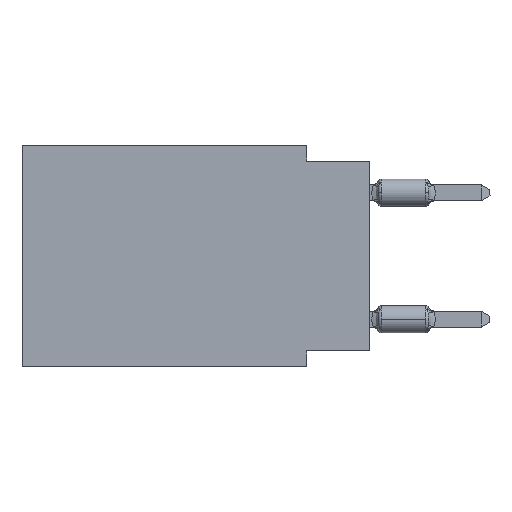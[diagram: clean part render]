
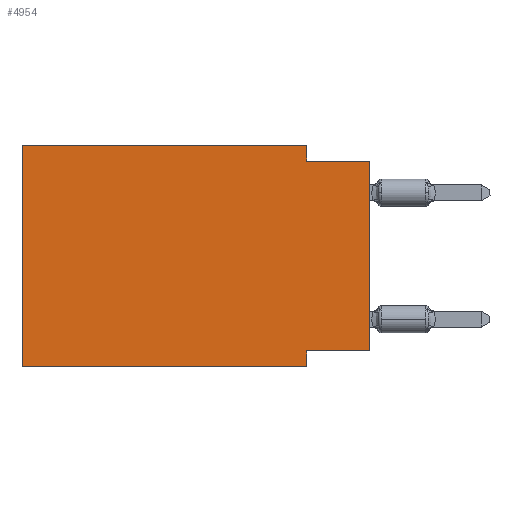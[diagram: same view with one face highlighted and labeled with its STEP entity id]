
A CAD part, left-side view. The second image highlights one B-rep face of the part: STEP entity #4954.
In plain terms, the highlighted planar face has unit normal (-1, 0, 0).
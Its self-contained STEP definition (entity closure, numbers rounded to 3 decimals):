
#300 = ORIENTED_EDGE ( 'NONE', *, *, #9761, .F. ) ;
#511 = CARTESIAN_POINT ( 'NONE',  ( 0., 2.54, 0. ) ) ;
#839 = ORIENTED_EDGE ( 'NONE', *, *, #12139, .T. ) ;
#884 = DIRECTION ( 'NONE',  ( 1., 0., 0. ) ) ;
#1540 = VECTOR ( 'NONE', #4809, 1000. ) ;
#1680 = ORIENTED_EDGE ( 'NONE', *, *, #12162, .F. ) ;
#1848 = PLANE ( 'NONE',  #8297 ) ;
#2168 = CARTESIAN_POINT ( 'NONE',  ( 0., 0., -8.255 ) ) ;
#2291 = VERTEX_POINT ( 'NONE', #4083 ) ;
#2313 = LINE ( 'NONE', #2168, #4158 ) ;
#2399 = DIRECTION ( 'NONE',  ( 0., 0., 1. ) ) ;
#2485 = DIRECTION ( 'NONE',  ( 0., -1., 0. ) ) ;
#2576 = LINE ( 'NONE', #3664, #7910 ) ;
#2777 = CARTESIAN_POINT ( 'NONE',  ( 0., 2.54, 0. ) ) ;
#3143 = VERTEX_POINT ( 'NONE', #5283 ) ;
#3512 = CARTESIAN_POINT ( 'NONE',  ( 0., 2.54, -8.89 ) ) ;
#3590 = EDGE_CURVE ( 'NONE', #2291, #4291, #6506, .T. ) ;
#3664 = CARTESIAN_POINT ( 'NONE',  ( 0., 13.97, -8.89 ) ) ;
#4083 = CARTESIAN_POINT ( 'NONE',  ( 0., 0., -8.255 ) ) ;
#4122 = VECTOR ( 'NONE', #11847, 1000. ) ;
#4158 = VECTOR ( 'NONE', #10649, 1000. ) ;
#4185 = ORIENTED_EDGE ( 'NONE', *, *, #3590, .T. ) ;
#4291 = VERTEX_POINT ( 'NONE', #11838 ) ;
#4340 = VECTOR ( 'NONE', #11898, 1000. ) ;
#4761 = CARTESIAN_POINT ( 'NONE',  ( 0., 2.54, -8.255 ) ) ;
#4797 = LINE ( 'NONE', #13117, #10544 ) ;
#4809 = DIRECTION ( 'NONE',  ( 0., 0., 1. ) ) ;
#4879 = VERTEX_POINT ( 'NONE', #11066 ) ;
#4954 = ADVANCED_FACE ( 'NONE', ( #13419 ), #1848, .F. ) ;
#5283 = CARTESIAN_POINT ( 'NONE',  ( 0., 13.97, -8.89 ) ) ;
#5302 = VERTEX_POINT ( 'NONE', #4761 ) ;
#5675 = CARTESIAN_POINT ( 'NONE',  ( 0., 0., -0.635 ) ) ;
#5985 = ORIENTED_EDGE ( 'NONE', *, *, #11480, .F. ) ;
#6180 = ORIENTED_EDGE ( 'NONE', *, *, #13039, .F. ) ;
#6506 = LINE ( 'NONE', #11755, #7008 ) ;
#6932 = LINE ( 'NONE', #8078, #1540 ) ;
#7008 = VECTOR ( 'NONE', #2399, 1000. ) ;
#7540 = EDGE_LOOP ( 'NONE', ( #4185, #11945, #1680, #6180, #12651, #839, #300, #5985 ) ) ;
#7745 = LINE ( 'NONE', #5675, #4340 ) ;
#7838 = DIRECTION ( 'NONE',  ( 0., -1., 0. ) ) ;
#7910 = VECTOR ( 'NONE', #7838, 1000. ) ;
#8078 = CARTESIAN_POINT ( 'NONE',  ( 0., 13.97, 0. ) ) ;
#8297 = AXIS2_PLACEMENT_3D ( 'NONE', #11452, #884, #13286 ) ;
#8632 = EDGE_CURVE ( 'NONE', #4879, #4291, #7745, .T. ) ;
#8642 = VERTEX_POINT ( 'NONE', #511 ) ;
#8775 = VECTOR ( 'NONE', #10984, 1000. ) ;
#8840 = LINE ( 'NONE', #3512, #4122 ) ;
#9761 = EDGE_CURVE ( 'NONE', #5302, #10036, #8840, .T. ) ;
#10036 = VERTEX_POINT ( 'NONE', #12565 ) ;
#10059 = CARTESIAN_POINT ( 'NONE',  ( 0., 13.97, 0. ) ) ;
#10544 = VECTOR ( 'NONE', #2485, 1000. ) ;
#10649 = DIRECTION ( 'NONE',  ( 0., 1., 0. ) ) ;
#10984 = DIRECTION ( 'NONE',  ( 0., 0., -1. ) ) ;
#11066 = CARTESIAN_POINT ( 'NONE',  ( 0., 2.54, -0.635 ) ) ;
#11110 = EDGE_CURVE ( 'NONE', #3143, #11897, #6932, .T. ) ;
#11452 = CARTESIAN_POINT ( 'NONE',  ( 0., 13.97, 0. ) ) ;
#11480 = EDGE_CURVE ( 'NONE', #2291, #5302, #2313, .T. ) ;
#11755 = CARTESIAN_POINT ( 'NONE',  ( 0., 0., 0. ) ) ;
#11838 = CARTESIAN_POINT ( 'NONE',  ( 0., 0., -0.635 ) ) ;
#11847 = DIRECTION ( 'NONE',  ( 0., 0., -1. ) ) ;
#11897 = VERTEX_POINT ( 'NONE', #10059 ) ;
#11898 = DIRECTION ( 'NONE',  ( 0., -1., 0. ) ) ;
#11945 = ORIENTED_EDGE ( 'NONE', *, *, #8632, .F. ) ;
#12139 = EDGE_CURVE ( 'NONE', #3143, #10036, #2576, .T. ) ;
#12162 = EDGE_CURVE ( 'NONE', #8642, #4879, #12190, .T. ) ;
#12190 = LINE ( 'NONE', #2777, #8775 ) ;
#12565 = CARTESIAN_POINT ( 'NONE',  ( 0., 2.54, -8.89 ) ) ;
#12651 = ORIENTED_EDGE ( 'NONE', *, *, #11110, .F. ) ;
#13039 = EDGE_CURVE ( 'NONE', #11897, #8642, #4797, .T. ) ;
#13117 = CARTESIAN_POINT ( 'NONE',  ( 0., 13.97, 0. ) ) ;
#13286 = DIRECTION ( 'NONE',  ( 0., 0., -1. ) ) ;
#13419 = FACE_OUTER_BOUND ( 'NONE', #7540, .T. ) ;
